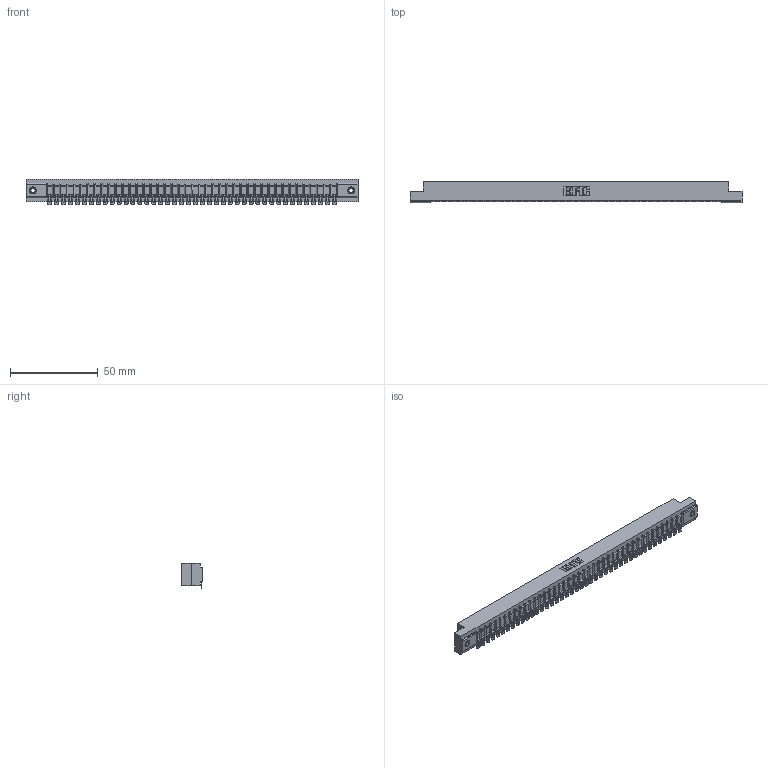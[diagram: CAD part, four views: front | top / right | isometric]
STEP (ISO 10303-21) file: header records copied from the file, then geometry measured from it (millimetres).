
FILE_DESCRIPTION (( 'STEP AP203' ), '1' );
FILE_NAME ('307-042-454-107.STEP', '2020-09-29T18:19:57', ( '' ), ( '' ), 'SwSTEP 2.0', 'SolidWorks 2020', '' );
FILE_SCHEMA (( 'CONFIG_CONTROL_DESIGN' ));
Length unit declared in the file: inch
Products named in the file (4): 307-042-454-107; 345-250-001_345-250-005-103; 307 Part_.156 Dia Mounting Holes; 307-290-002_554
Assembly tree (45 placements, depth 2):
  307-042-454-107
    307 Part_.156 Dia Mounting Holes
    307-290-002_554  x42
    345-250-001_345-250-005-103  x2
Bounding box: 189.43 x 12.01 x 14.52 mm (x, y, z)
Volume: 20273.4 mm3; surface area: 25685.1 mm2
Topology: 45 solids, 45 shells, 3623 faces, 11085 edges, 7266 vertices
Faces by surface type: plane 2034, cylinder 1487, sphere 86, cone 12, torus 4
Entity records: 38156 total; most frequent: CARTESIAN_POINT 6417, ORIENTED_EDGE 6400, DIRECTION 6250, EDGE_CURVE 3200, LINE 2444, VECTOR 2444, VERTEX_POINT 2070, AXIS2_PLACEMENT_3D 1903
